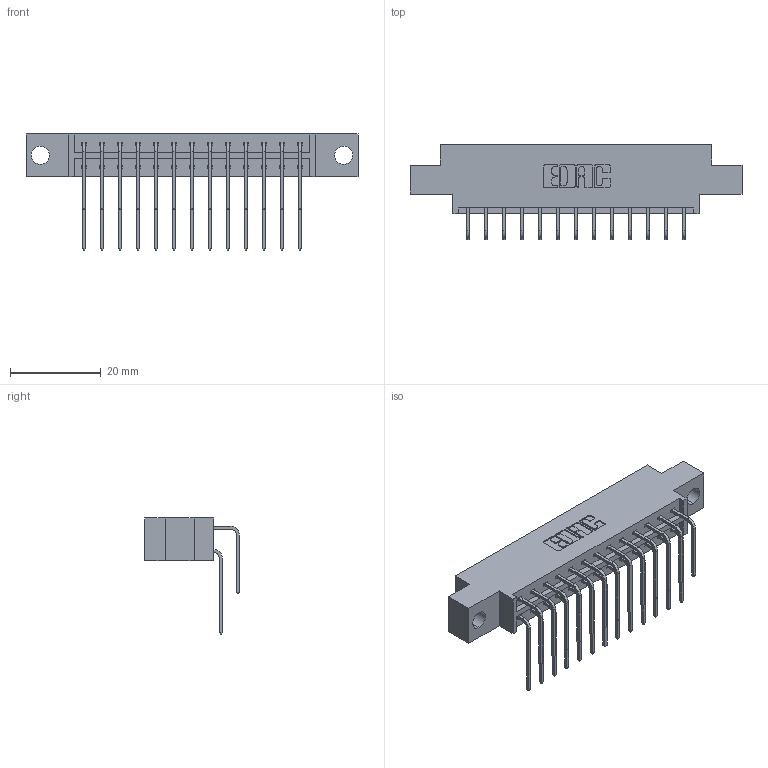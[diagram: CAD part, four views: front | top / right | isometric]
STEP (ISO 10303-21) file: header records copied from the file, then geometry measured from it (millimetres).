
FILE_DESCRIPTION (( 'STEP AP203' ), '1' );
FILE_NAME ('333-026-559-804.STEP', '2018-08-02T13:35:51', ( '' ), ( '' ), 'SwSTEP 2.0', 'SolidWorks 2016', '' );
FILE_SCHEMA (( 'CONFIG_CONTROL_DESIGN' ));
Length unit declared in the file: inch
Products named in the file (4): 333 Part_Offset - .156 Dia - TH; 345-292-001_558 559 Tail - 1; 345-292-001_559 Tail - 2; 333-026-559-804
Assembly tree (27 placements, depth 2):
  333-026-559-804
    333 Part_Offset - .156 Dia - TH
    345-292-001_558 559 Tail - 1  x13
    345-292-001_559 Tail - 2  x13
Bounding box: 73.05 x 20.9 x 25.53 mm (x, y, z)
Volume: 7021.2 mm3; surface area: 8756.5 mm2
Topology: 27 solids, 27 shells, 1522 faces, 4509 edges, 2970 vertices
Faces by surface type: plane 1062, cylinder 460
Entity records: 14033 total; most frequent: CARTESIAN_POINT 2413, ORIENTED_EDGE 2298, DIRECTION 2093, EDGE_CURVE 1149, VECTOR 981, LINE 981, VERTEX_POINT 762, AXIS2_PLACEMENT_3D 556
